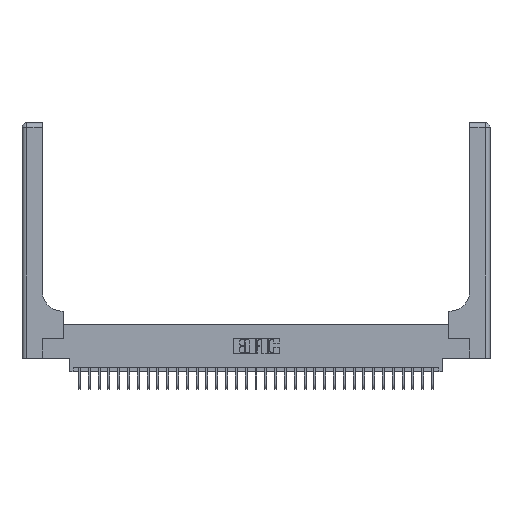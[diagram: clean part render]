
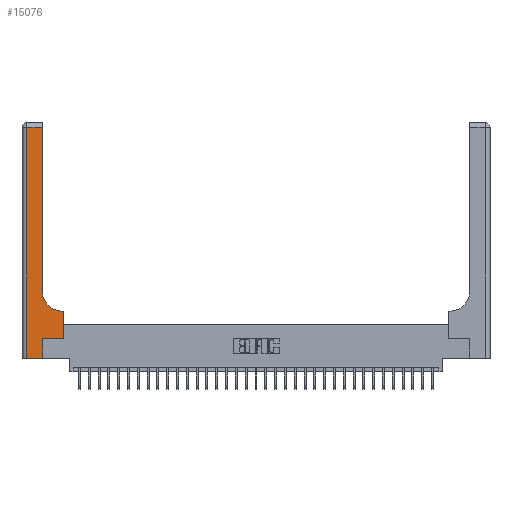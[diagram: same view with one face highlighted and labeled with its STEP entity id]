
A CAD part, top view. The second image highlights one B-rep face of the part: STEP entity #15076.
In plain terms, the highlighted planar face has unit normal (0, 0, 1).
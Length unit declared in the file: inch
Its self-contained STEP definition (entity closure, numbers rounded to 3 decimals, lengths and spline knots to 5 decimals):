
#102 = LINE ( 'NONE', #17663, #11731 ) ;
#966 = LINE ( 'NONE', #25911, #22713 ) ;
#972 = LINE ( 'NONE', #28686, #26332 ) ;
#1276 = DIRECTION ( 'NONE',  ( 0., 0., -1. ) ) ;
#1680 = ORIENTED_EDGE ( 'NONE', *, *, #28222, .T. ) ;
#2324 = CARTESIAN_POINT ( 'NONE',  ( 0.26, 2.94, 0.37 ) ) ;
#2527 = VECTOR ( 'NONE', #17158, 39.37008 ) ;
#2553 = CARTESIAN_POINT ( 'NONE',  ( 0.265, 0.25, 0.37 ) ) ;
#3232 = CARTESIAN_POINT ( 'NONE',  ( 0., 3., 0.37 ) ) ;
#3284 = DIRECTION ( 'NONE',  ( 0., -1., 0. ) ) ;
#3445 = DIRECTION ( 'NONE',  ( 1., 0., 0. ) ) ;
#4214 = ORIENTED_EDGE ( 'NONE', *, *, #12053, .T. ) ;
#4725 = CARTESIAN_POINT ( 'NONE',  ( 0.26, 0.85, 0.37 ) ) ;
#4915 = DIRECTION ( 'NONE',  ( 0., 1., 0. ) ) ;
#5646 = CARTESIAN_POINT ( 'NONE',  ( 0.06, 0., 0.37 ) ) ;
#6945 = ORIENTED_EDGE ( 'NONE', *, *, #19059, .T. ) ;
#7907 = ORIENTED_EDGE ( 'NONE', *, *, #22297, .T. ) ;
#8018 = VECTOR ( 'NONE', #29382, 39.37008 ) ;
#8399 = AXIS2_PLACEMENT_3D ( 'NONE', #24518, #22070, #32042 ) ;
#8870 = VERTEX_POINT ( 'NONE', #25684 ) ;
#9391 = LINE ( 'NONE', #19398, #8018 ) ;
#10633 = DIRECTION ( 'NONE',  ( -1., 0., 0. ) ) ;
#11731 = VECTOR ( 'NONE', #30261, 39.37008 ) ;
#12053 = EDGE_CURVE ( 'NONE', #32262, #16577, #966, .T. ) ;
#13296 = CARTESIAN_POINT ( 'NONE',  ( 0.06, 2.94, 0.37 ) ) ;
#13373 = EDGE_LOOP ( 'NONE', ( #28441, #1680, #32159, #4214, #30463, #7907, #6945, #19517, #26100 ) ) ;
#13462 = VERTEX_POINT ( 'NONE', #13296 ) ;
#13472 = CARTESIAN_POINT ( 'NONE',  ( 0.51, 0.6, 0.37 ) ) ;
#13556 = EDGE_CURVE ( 'NONE', #20651, #31596, #972, .T. ) ;
#14398 = CARTESIAN_POINT ( 'NONE',  ( 0.265, 0., 0.37 ) ) ;
#15076 = ADVANCED_FACE ( 'NONE', ( #26194 ), #23915, .F. ) ;
#16470 = EDGE_CURVE ( 'NONE', #13462, #32262, #21008, .T. ) ;
#16523 = EDGE_CURVE ( 'NONE', #16577, #27015, #27651, .T. ) ;
#16577 = VERTEX_POINT ( 'NONE', #32247 ) ;
#16662 = VERTEX_POINT ( 'NONE', #30904 ) ;
#17158 = DIRECTION ( 'NONE',  ( 1., 0., 0. ) ) ;
#17663 = CARTESIAN_POINT ( 'NONE',  ( 0., 2.94, 0.37 ) ) ;
#18722 = AXIS2_PLACEMENT_3D ( 'NONE', #3232, #1276, #10633 ) ;
#19059 = EDGE_CURVE ( 'NONE', #16662, #8870, #21842, .T. ) ;
#19398 = CARTESIAN_POINT ( 'NONE',  ( 0.26, 0.6, 0.37 ) ) ;
#19517 = ORIENTED_EDGE ( 'NONE', *, *, #27864, .T. ) ;
#19648 = DIRECTION ( 'NONE',  ( 0., 1., 0. ) ) ;
#20651 = VERTEX_POINT ( 'NONE', #4725 ) ;
#21008 = LINE ( 'NONE', #25757, #25410 ) ;
#21842 = LINE ( 'NONE', #27388, #25002 ) ;
#22070 = DIRECTION ( 'NONE',  ( 0., 0., -1. ) ) ;
#22297 = EDGE_CURVE ( 'NONE', #27015, #16662, #27324, .T. ) ;
#22713 = VECTOR ( 'NONE', #3445, 39.37008 ) ;
#23863 = VECTOR ( 'NONE', #19648, 39.37008 ) ;
#23915 = PLANE ( 'NONE',  #18722 ) ;
#24251 = CARTESIAN_POINT ( 'NONE',  ( 0.265, 0.25, 0.37 ) ) ;
#24501 = EDGE_CURVE ( 'NONE', #25300, #20651, #31420, .T. ) ;
#24518 = CARTESIAN_POINT ( 'NONE',  ( 0.51, 0.85, 0.37 ) ) ;
#25002 = VECTOR ( 'NONE', #4915, 39.37008 ) ;
#25300 = VERTEX_POINT ( 'NONE', #13472 ) ;
#25410 = VECTOR ( 'NONE', #3284, 39.37008 ) ;
#25684 = CARTESIAN_POINT ( 'NONE',  ( 0.528, 0.6, 0.37 ) ) ;
#25757 = CARTESIAN_POINT ( 'NONE',  ( 0.06, 3., 0.37 ) ) ;
#25911 = CARTESIAN_POINT ( 'NONE',  ( 0., 0., 0.37 ) ) ;
#26100 = ORIENTED_EDGE ( 'NONE', *, *, #24501, .T. ) ;
#26194 = FACE_OUTER_BOUND ( 'NONE', #13373, .T. ) ;
#26332 = VECTOR ( 'NONE', #30973, 39.37008 ) ;
#27015 = VERTEX_POINT ( 'NONE', #24251 ) ;
#27324 = LINE ( 'NONE', #2553, #2527 ) ;
#27388 = CARTESIAN_POINT ( 'NONE',  ( 0.528, 0.25, 0.37 ) ) ;
#27651 = LINE ( 'NONE', #14398, #23863 ) ;
#27864 = EDGE_CURVE ( 'NONE', #8870, #25300, #9391, .T. ) ;
#28222 = EDGE_CURVE ( 'NONE', #31596, #13462, #102, .T. ) ;
#28441 = ORIENTED_EDGE ( 'NONE', *, *, #13556, .T. ) ;
#28686 = CARTESIAN_POINT ( 'NONE',  ( 0.26, 3., 0.37 ) ) ;
#29382 = DIRECTION ( 'NONE',  ( -1., 0., 0. ) ) ;
#30261 = DIRECTION ( 'NONE',  ( -1., 0., 0. ) ) ;
#30463 = ORIENTED_EDGE ( 'NONE', *, *, #16523, .T. ) ;
#30904 = CARTESIAN_POINT ( 'NONE',  ( 0.528, 0.25, 0.37 ) ) ;
#30973 = DIRECTION ( 'NONE',  ( 0., 1., 0. ) ) ;
#31420 = CIRCLE ( 'NONE', #8399, 0.25 ) ;
#31596 = VERTEX_POINT ( 'NONE', #2324 ) ;
#32042 = DIRECTION ( 'NONE',  ( 1., 0., 0. ) ) ;
#32159 = ORIENTED_EDGE ( 'NONE', *, *, #16470, .T. ) ;
#32247 = CARTESIAN_POINT ( 'NONE',  ( 0.265, 0., 0.37 ) ) ;
#32262 = VERTEX_POINT ( 'NONE', #5646 ) ;
